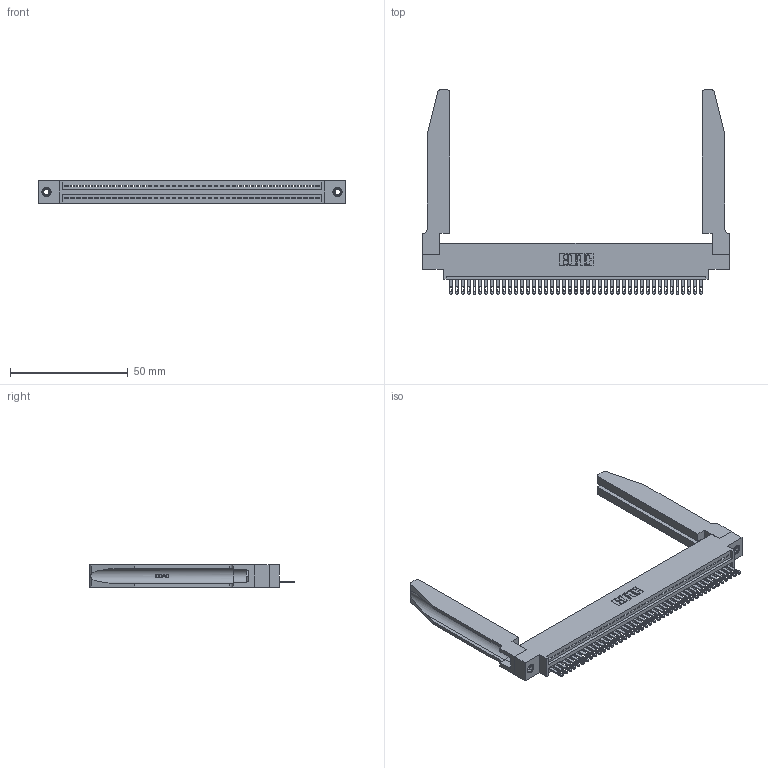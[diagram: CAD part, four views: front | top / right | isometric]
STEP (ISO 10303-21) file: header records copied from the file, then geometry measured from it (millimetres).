
FILE_DESCRIPTION (( 'STEP AP203' ), '1' );
FILE_NAME ('345-043-500-678.STEP', '2019-10-08T15:43:54', ( '' ), ( '' ), 'SwSTEP 2.0', 'SolidWorks 2016', '' );
FILE_SCHEMA (( 'CONFIG_CONTROL_DESIGN' ));
Length unit declared in the file: inch
Products named in the file (5): 345-250-001_345-250-001-102; 345-220-078_345-220-078; 345-292-001_345-293-100; 345-043-500-678; 345 Part_0.170 Offset - 0.156 Dia-TH
Assembly tree (48 placements, depth 2):
  345-043-500-678
    345 Part_0.170 Offset - 0.156 Dia-TH
    345-292-001_345-293-100  x43
    345-250-001_345-250-001-102  x2
    345-220-078_345-220-078  x2
Bounding box: 130.45 x 86.79 x 9.4 mm (x, y, z)
Volume: 20082.6 mm3; surface area: 23444 mm2
Topology: 48 solids, 48 shells, 2686 faces, 8185 edges, 5446 vertices
Faces by surface type: plane 1688, cylinder 946, bspline 36, cone 12, torus 4
Entity records: 37030 total; most frequent: CARTESIAN_POINT 7312, ORIENTED_EDGE 6186, DIRECTION 5393, EDGE_CURVE 3093, VECTOR 2691, LINE 2691, VERTEX_POINT 2056, AXIS2_PLACEMENT_3D 1351
